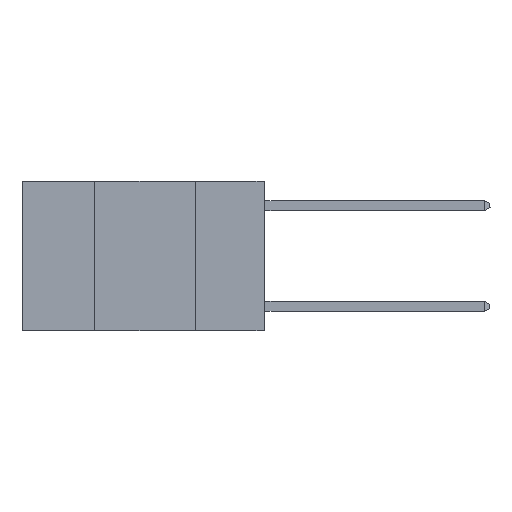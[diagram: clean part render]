
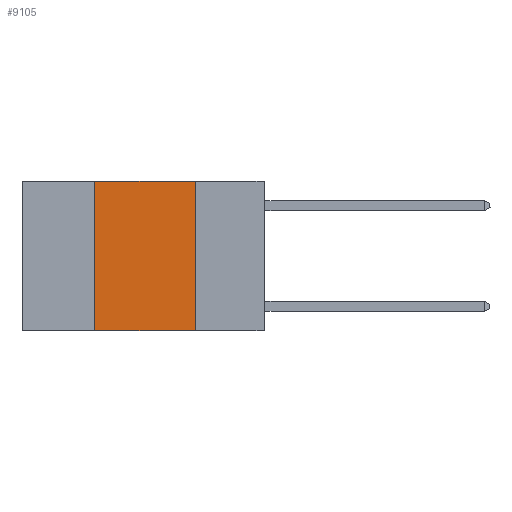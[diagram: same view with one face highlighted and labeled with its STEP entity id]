
A CAD part, left-side view. The second image highlights one B-rep face of the part: STEP entity #9105.
In plain terms, the highlighted planar face has unit normal (-1, 0, 0).
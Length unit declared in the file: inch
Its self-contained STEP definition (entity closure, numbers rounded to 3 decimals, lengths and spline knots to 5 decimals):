
#207 = LINE ( 'NONE', #555, #6768 ) ;
#376 = FACE_OUTER_BOUND ( 'NONE', #1422, .T. ) ;
#534 = LINE ( 'NONE', #8915, #9486 ) ;
#555 = CARTESIAN_POINT ( 'NONE',  ( 0., 0.17, 0. ) ) ;
#606 = DIRECTION ( 'NONE',  ( 1., 0., 0. ) ) ;
#715 = EDGE_CURVE ( 'NONE', #3485, #5308, #6049, .T. ) ;
#1422 = EDGE_LOOP ( 'NONE', ( #4414, #4416, #4492, #4651 ) ) ;
#2400 = VECTOR ( 'NONE', #5414, 39.37008 ) ;
#2664 = EDGE_CURVE ( 'NONE', #6983, #7020, #534, .T. ) ;
#2880 = DIRECTION ( 'NONE',  ( 0., -1., 0. ) ) ;
#3292 = PLANE ( 'NONE',  #6695 ) ;
#3485 = VERTEX_POINT ( 'NONE', #5824 ) ;
#4099 = EDGE_CURVE ( 'NONE', #5308, #7020, #207, .T. ) ;
#4414 = ORIENTED_EDGE ( 'NONE', *, *, #4099, .F. ) ;
#4416 = ORIENTED_EDGE ( 'NONE', *, *, #715, .F. ) ;
#4492 = ORIENTED_EDGE ( 'NONE', *, *, #8109, .F. ) ;
#4548 = CARTESIAN_POINT ( 'NONE',  ( 0., 0.42, 0. ) ) ;
#4651 = ORIENTED_EDGE ( 'NONE', *, *, #2664, .T. ) ;
#4766 = CARTESIAN_POINT ( 'NONE',  ( 0., 0.17, -0.37 ) ) ;
#5046 = CARTESIAN_POINT ( 'NONE',  ( 0., 0.17, 0. ) ) ;
#5308 = VERTEX_POINT ( 'NONE', #5046 ) ;
#5414 = DIRECTION ( 'NONE',  ( 0., 0., 1. ) ) ;
#5507 = VECTOR ( 'NONE', #8188, 39.37008 ) ;
#5626 = CARTESIAN_POINT ( 'NONE',  ( 0., 0.42, -0.37 ) ) ;
#5667 = CARTESIAN_POINT ( 'NONE',  ( 0., 0.6, 0. ) ) ;
#5824 = CARTESIAN_POINT ( 'NONE',  ( 0., 0.42, 0. ) ) ;
#6049 = LINE ( 'NONE', #5667, #5507 ) ;
#6695 = AXIS2_PLACEMENT_3D ( 'NONE', #10083, #606, #6836 ) ;
#6768 = VECTOR ( 'NONE', #6784, 39.37008 ) ;
#6784 = DIRECTION ( 'NONE',  ( 0., 0., -1. ) ) ;
#6836 = DIRECTION ( 'NONE',  ( 0., 0., -1. ) ) ;
#6983 = VERTEX_POINT ( 'NONE', #5626 ) ;
#7020 = VERTEX_POINT ( 'NONE', #4766 ) ;
#8109 = EDGE_CURVE ( 'NONE', #6983, #3485, #9242, .T. ) ;
#8188 = DIRECTION ( 'NONE',  ( 0., -1., 0. ) ) ;
#8915 = CARTESIAN_POINT ( 'NONE',  ( 0., 0.6, -0.37 ) ) ;
#9105 = ADVANCED_FACE ( 'NONE', ( #376 ), #3292, .F. ) ;
#9242 = LINE ( 'NONE', #4548, #2400 ) ;
#9486 = VECTOR ( 'NONE', #2880, 39.37008 ) ;
#10083 = CARTESIAN_POINT ( 'NONE',  ( 0., 0.6, 0. ) ) ;
